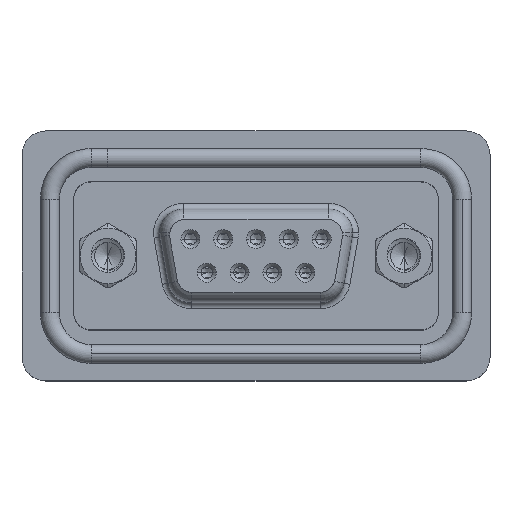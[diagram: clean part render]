
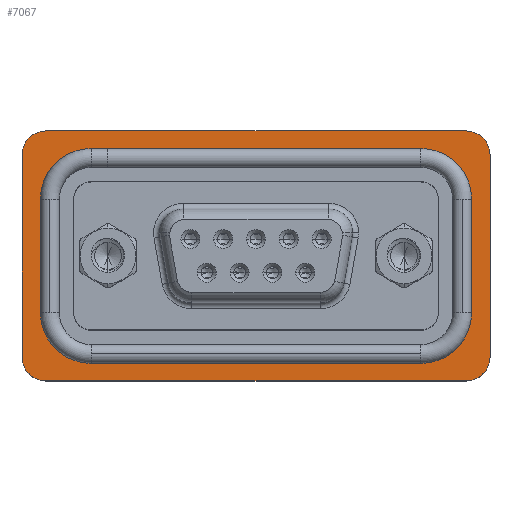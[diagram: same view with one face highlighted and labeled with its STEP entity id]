
A CAD part, top view. The second image highlights one B-rep face of the part: STEP entity #7067.
In plain terms, the highlighted planar face has unit normal (0, 0, 1).
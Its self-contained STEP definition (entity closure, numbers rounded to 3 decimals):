
#35 = ORIENTED_EDGE ( 'NONE', *, *, #4100, .F. ) ;
#55 = VERTEX_POINT ( 'NONE', #15291 ) ;
#109 = DIRECTION ( 'NONE',  ( 0., -1., 0. ) ) ;
#320 = EDGE_CURVE ( 'NONE', #12741, #55, #4344, .T. ) ;
#663 = DIRECTION ( 'NONE',  ( 1., 0., 0. ) ) ;
#817 = CIRCLE ( 'NONE', #5537, 2. ) ;
#1107 = EDGE_CURVE ( 'NONE', #3882, #22483, #11854, .T. ) ;
#1180 = EDGE_CURVE ( 'NONE', #15822, #3882, #1897, .T. ) ;
#1897 = LINE ( 'NONE', #7073, #17292 ) ;
#1962 = AXIS2_PLACEMENT_3D ( 'NONE', #9838, #6621, #22435 ) ;
#2135 = CARTESIAN_POINT ( 'NONE',  ( -1.41, -4.775, 0.4 ) ) ;
#2358 = DIRECTION ( 'NONE',  ( 0., 0., 1. ) ) ;
#2662 = DIRECTION ( 'NONE',  ( 1., 0., 0. ) ) ;
#2901 = CIRCLE ( 'NONE', #14624, 2. ) ;
#3536 = CARTESIAN_POINT ( 'NONE',  ( -5.71, 4.775, 0.4 ) ) ;
#3639 = EDGE_CURVE ( 'NONE', #16409, #4053, #10663, .T. ) ;
#3882 = VERTEX_POINT ( 'NONE', #13729 ) ;
#4053 = VERTEX_POINT ( 'NONE', #22666 ) ;
#4100 = EDGE_CURVE ( 'NONE', #13666, #18637, #17483, .T. ) ;
#4106 = CARTESIAN_POINT ( 'NONE',  ( 30.25, -8.55, 0.4 ) ) ;
#4307 = DIRECTION ( 'NONE',  ( 1., 0., 0. ) ) ;
#4344 = LINE ( 'NONE', #21995, #10539 ) ;
#4500 = DIRECTION ( 'NONE',  ( 0., 1., 0. ) ) ;
#4640 = CARTESIAN_POINT ( 'NONE',  ( -5.26, -8.55, 0.4 ) ) ;
#5002 = FACE_BOUND ( 'NONE', #8496, .T. ) ;
#5521 = CARTESIAN_POINT ( 'NONE',  ( -5.26, -10.55, 0.4 ) ) ;
#5537 = AXIS2_PLACEMENT_3D ( 'NONE', #4640, #9941, #13133 ) ;
#6005 = VERTEX_POINT ( 'NONE', #12444 ) ;
#6048 = DIRECTION ( 'NONE',  ( 1., 0., 0. ) ) ;
#6064 = VECTOR ( 'NONE', #10632, 1000. ) ;
#6113 = EDGE_CURVE ( 'NONE', #18117, #17061, #16897, .T. ) ;
#6621 = DIRECTION ( 'NONE',  ( 0., 0., 1. ) ) ;
#6830 = EDGE_CURVE ( 'NONE', #55, #15822, #9076, .T. ) ;
#6885 = CIRCLE ( 'NONE', #13458, 4.3 ) ;
#6933 = ORIENTED_EDGE ( 'NONE', *, *, #320, .T. ) ;
#6983 = CARTESIAN_POINT ( 'NONE',  ( -1.41, 4.775, 0.4 ) ) ;
#7067 = ADVANCED_FACE ( 'NONE', ( #5002, #22543 ), #19425, .T. ) ;
#7073 = CARTESIAN_POINT ( 'NONE',  ( 30.25, 10.55, 0.4 ) ) ;
#7301 = CARTESIAN_POINT ( 'NONE',  ( 26.4, 9.075, 0.4 ) ) ;
#7655 = VERTEX_POINT ( 'NONE', #5521 ) ;
#7894 = CARTESIAN_POINT ( 'NONE',  ( 30.25, -10.55, 0.4 ) ) ;
#7961 = VECTOR ( 'NONE', #11297, 1000. ) ;
#8009 = CIRCLE ( 'NONE', #21163, 4.3 ) ;
#8161 = AXIS2_PLACEMENT_3D ( 'NONE', #6983, #22677, #13965 ) ;
#8162 = EDGE_CURVE ( 'NONE', #15264, #13666, #6885, .T. ) ;
#8496 = EDGE_LOOP ( 'NONE', ( #20333, #19627, #8720, #12664, #21141, #13132, #16558, #35 ) ) ;
#8720 = ORIENTED_EDGE ( 'NONE', *, *, #20294, .F. ) ;
#8725 = ORIENTED_EDGE ( 'NONE', *, *, #13072, .T. ) ;
#8830 = EDGE_CURVE ( 'NONE', #6005, #15264, #18594, .T. ) ;
#8876 = CIRCLE ( 'NONE', #8161, 4.3 ) ;
#9076 = CIRCLE ( 'NONE', #18945, 2. ) ;
#9423 = CARTESIAN_POINT ( 'NONE',  ( -5.71, 4.775, 0.4 ) ) ;
#9488 = CARTESIAN_POINT ( 'NONE',  ( 30.25, 8.55, 0.4 ) ) ;
#9615 = CARTESIAN_POINT ( 'NONE',  ( -7.26, 8.55, 0.4 ) ) ;
#9678 = ORIENTED_EDGE ( 'NONE', *, *, #6830, .T. ) ;
#9809 = CARTESIAN_POINT ( 'NONE',  ( -1.41, -9.075, 0.4 ) ) ;
#9827 = VECTOR ( 'NONE', #4500, 1000. ) ;
#9838 = CARTESIAN_POINT ( 'NONE',  ( -5.26, 8.55, 0.4 ) ) ;
#9941 = DIRECTION ( 'NONE',  ( 0., 0., 1. ) ) ;
#10135 = EDGE_CURVE ( 'NONE', #15908, #12741, #2901, .T. ) ;
#10205 = CARTESIAN_POINT ( 'NONE',  ( 30.7, 4.775, 0.4 ) ) ;
#10539 = VECTOR ( 'NONE', #16072, 1000. ) ;
#10614 = CARTESIAN_POINT ( 'NONE',  ( 32.25, -8.55, 0.4 ) ) ;
#10632 = DIRECTION ( 'NONE',  ( -1., 0., 0. ) ) ;
#10663 = LINE ( 'NONE', #3536, #12622 ) ;
#10743 = DIRECTION ( 'NONE',  ( 0., 0., 1. ) ) ;
#10970 = DIRECTION ( 'NONE',  ( 1., 0., 0. ) ) ;
#11110 = DIRECTION ( 'NONE',  ( 0., 0., 1. ) ) ;
#11151 = CARTESIAN_POINT ( 'NONE',  ( 26.4, -4.775, 0.4 ) ) ;
#11297 = DIRECTION ( 'NONE',  ( 1., 0., 0. ) ) ;
#11334 = DIRECTION ( 'NONE',  ( 1., 0., 0. ) ) ;
#11426 = VECTOR ( 'NONE', #663, 1000. ) ;
#11527 = CARTESIAN_POINT ( 'NONE',  ( -1.41, -9.075, 0.4 ) ) ;
#11854 = CIRCLE ( 'NONE', #1962, 2. ) ;
#11910 = EDGE_CURVE ( 'NONE', #22483, #20928, #17194, .T. ) ;
#11982 = AXIS2_PLACEMENT_3D ( 'NONE', #20815, #10743, #13723 ) ;
#12234 = EDGE_LOOP ( 'NONE', ( #9678, #13397, #20173, #14441, #21812, #8725, #19176, #6933 ) ) ;
#12444 = CARTESIAN_POINT ( 'NONE',  ( 30.7, -4.775, 0.4 ) ) ;
#12622 = VECTOR ( 'NONE', #109, 1000. ) ;
#12664 = ORIENTED_EDGE ( 'NONE', *, *, #6113, .F. ) ;
#12741 = VERTEX_POINT ( 'NONE', #10614 ) ;
#12985 = DIRECTION ( 'NONE',  ( 0., -1., 0. ) ) ;
#13072 = EDGE_CURVE ( 'NONE', #7655, #15908, #19913, .T. ) ;
#13132 = ORIENTED_EDGE ( 'NONE', *, *, #3639, .F. ) ;
#13133 = DIRECTION ( 'NONE',  ( -1., 0., 0. ) ) ;
#13213 = CARTESIAN_POINT ( 'NONE',  ( 30.7, -4.775, 0.4 ) ) ;
#13397 = ORIENTED_EDGE ( 'NONE', *, *, #1180, .T. ) ;
#13458 = AXIS2_PLACEMENT_3D ( 'NONE', #18161, #2358, #10970 ) ;
#13575 = EDGE_CURVE ( 'NONE', #4053, #18117, #15102, .T. ) ;
#13666 = VERTEX_POINT ( 'NONE', #21275 ) ;
#13682 = EDGE_CURVE ( 'NONE', #20928, #7655, #817, .T. ) ;
#13723 = DIRECTION ( 'NONE',  ( 1., 0., 0. ) ) ;
#13729 = CARTESIAN_POINT ( 'NONE',  ( -5.26, 10.55, 0.4 ) ) ;
#13965 = DIRECTION ( 'NONE',  ( 1., 0., 0. ) ) ;
#14441 = ORIENTED_EDGE ( 'NONE', *, *, #11910, .T. ) ;
#14624 = AXIS2_PLACEMENT_3D ( 'NONE', #4106, #11110, #11334 ) ;
#15034 = DIRECTION ( 'NONE',  ( 0., 0., 1. ) ) ;
#15102 = CIRCLE ( 'NONE', #20945, 4.3 ) ;
#15264 = VERTEX_POINT ( 'NONE', #10205 ) ;
#15291 = CARTESIAN_POINT ( 'NONE',  ( 32.25, 8.55, 0.4 ) ) ;
#15401 = EDGE_CURVE ( 'NONE', #18637, #16409, #8876, .T. ) ;
#15822 = VERTEX_POINT ( 'NONE', #19528 ) ;
#15908 = VERTEX_POINT ( 'NONE', #21707 ) ;
#16072 = DIRECTION ( 'NONE',  ( 0., 1., 0. ) ) ;
#16409 = VERTEX_POINT ( 'NONE', #9423 ) ;
#16456 = DIRECTION ( 'NONE',  ( 0., 0., 1. ) ) ;
#16558 = ORIENTED_EDGE ( 'NONE', *, *, #15401, .F. ) ;
#16645 = CARTESIAN_POINT ( 'NONE',  ( -7.26, -8.55, 0.4 ) ) ;
#16897 = LINE ( 'NONE', #9809, #7961 ) ;
#17061 = VERTEX_POINT ( 'NONE', #21093 ) ;
#17194 = LINE ( 'NONE', #16645, #17965 ) ;
#17292 = VECTOR ( 'NONE', #17471, 1000. ) ;
#17471 = DIRECTION ( 'NONE',  ( -1., 0., 0. ) ) ;
#17483 = LINE ( 'NONE', #7301, #6064 ) ;
#17926 = CARTESIAN_POINT ( 'NONE',  ( -7.26, -8.55, 0.4 ) ) ;
#17965 = VECTOR ( 'NONE', #12985, 1000. ) ;
#18117 = VERTEX_POINT ( 'NONE', #11527 ) ;
#18161 = CARTESIAN_POINT ( 'NONE',  ( 26.4, 4.775, 0.4 ) ) ;
#18594 = LINE ( 'NONE', #13213, #9827 ) ;
#18637 = VERTEX_POINT ( 'NONE', #21072 ) ;
#18945 = AXIS2_PLACEMENT_3D ( 'NONE', #9488, #21743, #6048 ) ;
#19176 = ORIENTED_EDGE ( 'NONE', *, *, #10135, .T. ) ;
#19425 = PLANE ( 'NONE',  #11982 ) ;
#19528 = CARTESIAN_POINT ( 'NONE',  ( 30.25, 10.55, 0.4 ) ) ;
#19627 = ORIENTED_EDGE ( 'NONE', *, *, #8830, .F. ) ;
#19913 = LINE ( 'NONE', #7894, #11426 ) ;
#20173 = ORIENTED_EDGE ( 'NONE', *, *, #1107, .T. ) ;
#20294 = EDGE_CURVE ( 'NONE', #17061, #6005, #8009, .T. ) ;
#20333 = ORIENTED_EDGE ( 'NONE', *, *, #8162, .F. ) ;
#20815 = CARTESIAN_POINT ( 'NONE',  ( 30.25, 8.55, 0.4 ) ) ;
#20928 = VERTEX_POINT ( 'NONE', #17926 ) ;
#20945 = AXIS2_PLACEMENT_3D ( 'NONE', #2135, #16456, #4307 ) ;
#21072 = CARTESIAN_POINT ( 'NONE',  ( -1.41, 9.075, 0.4 ) ) ;
#21093 = CARTESIAN_POINT ( 'NONE',  ( 26.4, -9.075, 0.4 ) ) ;
#21141 = ORIENTED_EDGE ( 'NONE', *, *, #13575, .F. ) ;
#21163 = AXIS2_PLACEMENT_3D ( 'NONE', #11151, #15034, #2662 ) ;
#21275 = CARTESIAN_POINT ( 'NONE',  ( 26.4, 9.075, 0.4 ) ) ;
#21707 = CARTESIAN_POINT ( 'NONE',  ( 30.25, -10.55, 0.4 ) ) ;
#21743 = DIRECTION ( 'NONE',  ( 0., 0., 1. ) ) ;
#21812 = ORIENTED_EDGE ( 'NONE', *, *, #13682, .T. ) ;
#21995 = CARTESIAN_POINT ( 'NONE',  ( 32.25, -8.55, 0.4 ) ) ;
#22435 = DIRECTION ( 'NONE',  ( 1., 0., 0. ) ) ;
#22483 = VERTEX_POINT ( 'NONE', #9615 ) ;
#22543 = FACE_OUTER_BOUND ( 'NONE', #12234, .T. ) ;
#22666 = CARTESIAN_POINT ( 'NONE',  ( -5.71, -4.775, 0.4 ) ) ;
#22677 = DIRECTION ( 'NONE',  ( 0., 0., 1. ) ) ;
